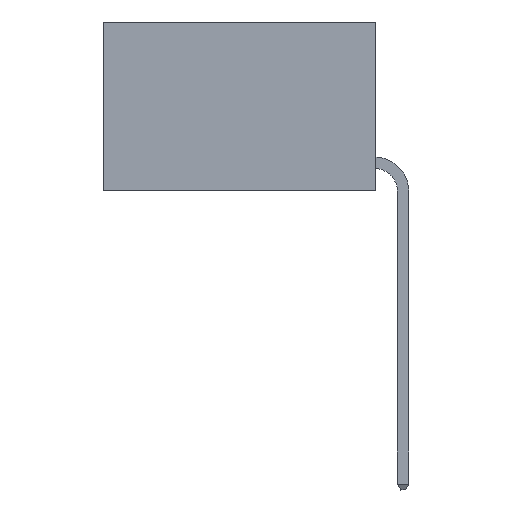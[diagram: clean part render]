
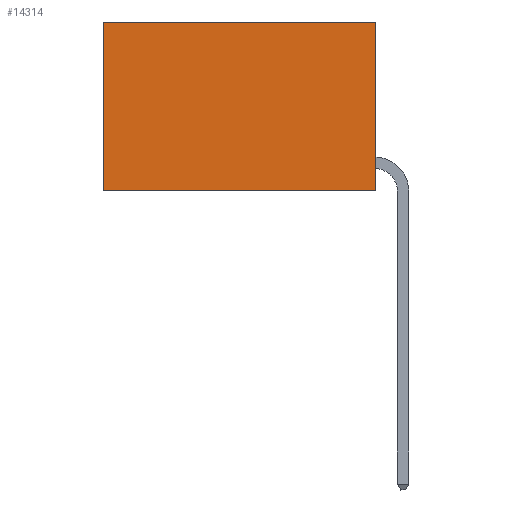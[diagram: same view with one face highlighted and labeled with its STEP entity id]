
A CAD part, left-side view. The second image highlights one B-rep face of the part: STEP entity #14314.
In plain terms, the highlighted planar face has unit normal (-1, 0, 0).
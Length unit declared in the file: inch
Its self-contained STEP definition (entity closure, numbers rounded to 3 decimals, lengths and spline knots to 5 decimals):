
#47 = CARTESIAN_POINT ( 'NONE',  ( 0.2625, 0., 0. ) ) ;
#534 = ORIENTED_EDGE ( 'NONE', *, *, #15752, .F. ) ;
#744 = DIRECTION ( 'NONE',  ( 0., 0., -1. ) ) ;
#831 = PLANE ( 'NONE',  #7973 ) ;
#1217 = CARTESIAN_POINT ( 'NONE',  ( 0.2625, 0., -0.37 ) ) ;
#1419 = VERTEX_POINT ( 'NONE', #3289 ) ;
#1953 = FACE_OUTER_BOUND ( 'NONE', #13151, .T. ) ;
#2089 = ORIENTED_EDGE ( 'NONE', *, *, #17146, .F. ) ;
#2612 = DIRECTION ( 'NONE',  ( 0., 0., -1. ) ) ;
#3289 = CARTESIAN_POINT ( 'NONE',  ( 0.2625, 0.6, 0. ) ) ;
#3476 = CARTESIAN_POINT ( 'NONE',  ( 0.2625, 0., -0.37 ) ) ;
#3557 = ORIENTED_EDGE ( 'NONE', *, *, #10395, .T. ) ;
#3778 = DIRECTION ( 'NONE',  ( 0., 0., -1. ) ) ;
#3976 = VECTOR ( 'NONE', #14485, 39.37008 ) ;
#5133 = CARTESIAN_POINT ( 'NONE',  ( 0.2625, 0., 0. ) ) ;
#5843 = VECTOR ( 'NONE', #744, 39.37008 ) ;
#6061 = CARTESIAN_POINT ( 'NONE',  ( 0.2625, 0., 0. ) ) ;
#6733 = VERTEX_POINT ( 'NONE', #47 ) ;
#6880 = VERTEX_POINT ( 'NONE', #9522 ) ;
#7346 = LINE ( 'NONE', #6061, #15169 ) ;
#7973 = AXIS2_PLACEMENT_3D ( 'NONE', #11150, #12648, #3778 ) ;
#8241 = VERTEX_POINT ( 'NONE', #3476 ) ;
#9522 = CARTESIAN_POINT ( 'NONE',  ( 0.2625, 0.6, -0.37 ) ) ;
#10395 = EDGE_CURVE ( 'NONE', #6733, #1419, #7346, .T. ) ;
#10457 = ORIENTED_EDGE ( 'NONE', *, *, #18584, .T. ) ;
#11150 = CARTESIAN_POINT ( 'NONE',  ( 0.2625, 0., 0. ) ) ;
#11480 = CARTESIAN_POINT ( 'NONE',  ( 0.2625, 0.6, 0. ) ) ;
#11848 = LINE ( 'NONE', #1217, #3976 ) ;
#12648 = DIRECTION ( 'NONE',  ( 1., 0., 0. ) ) ;
#13151 = EDGE_LOOP ( 'NONE', ( #10457, #534, #2089, #3557 ) ) ;
#13637 = LINE ( 'NONE', #5133, #5843 ) ;
#13956 = LINE ( 'NONE', #11480, #17876 ) ;
#14314 = ADVANCED_FACE ( 'NONE', ( #1953 ), #831, .F. ) ;
#14485 = DIRECTION ( 'NONE',  ( 0., 1., 0. ) ) ;
#15169 = VECTOR ( 'NONE', #16320, 39.37008 ) ;
#15752 = EDGE_CURVE ( 'NONE', #8241, #6880, #11848, .T. ) ;
#16320 = DIRECTION ( 'NONE',  ( 0., 1., 0. ) ) ;
#17146 = EDGE_CURVE ( 'NONE', #6733, #8241, #13637, .T. ) ;
#17876 = VECTOR ( 'NONE', #2612, 39.37008 ) ;
#18584 = EDGE_CURVE ( 'NONE', #1419, #6880, #13956, .T. ) ;
